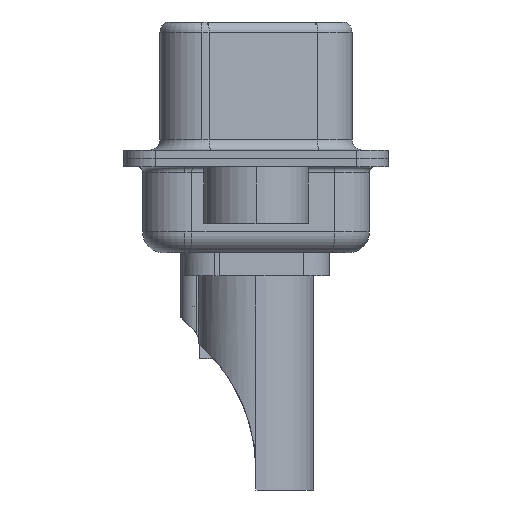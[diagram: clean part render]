
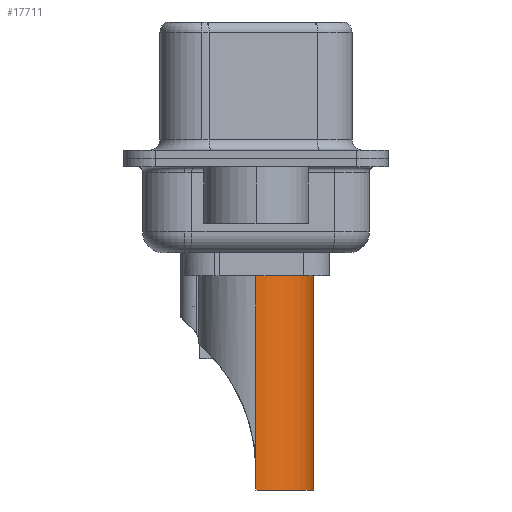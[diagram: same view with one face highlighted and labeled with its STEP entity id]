
A CAD part, left-side view. The second image highlights one B-rep face of the part: STEP entity #17711.
In plain terms, the highlighted cylindrical face has radius 2.75 mm (diameter 5.5 mm), a partial arc.
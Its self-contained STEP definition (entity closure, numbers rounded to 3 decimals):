
#143 = VECTOR ( 'NONE', #11961, 1000. ) ;
#347 = LINE ( 'NONE', #14707, #5019 ) ;
#400 = CARTESIAN_POINT ( 'NONE',  ( 2.75, 0., -8.7 ) ) ;
#703 = VECTOR ( 'NONE', #10427, 1000. ) ;
#766 = CARTESIAN_POINT ( 'NONE',  ( 2.75, 0., 1.5 ) ) ;
#983 = CARTESIAN_POINT ( 'NONE',  ( -2.75, 0., -8.7 ) ) ;
#1158 = CARTESIAN_POINT ( 'NONE',  ( -2.75, 0., 1.5 ) ) ;
#1320 = CARTESIAN_POINT ( 'NONE',  ( 2.75, 0., -7.764 ) ) ;
#1460 = DIRECTION ( 'NONE',  ( 1., 0., 0. ) ) ;
#2112 = VERTEX_POINT ( 'NONE', #766 ) ;
#2835 = VERTEX_POINT ( 'NONE', #983 ) ;
#2941 = LINE ( 'NONE', #4782, #13499 ) ;
#3705 = CYLINDRICAL_SURFACE ( 'NONE', #5382, 2.75 ) ;
#4361 = DIRECTION ( 'NONE',  ( 0., 0., 1. ) ) ;
#4432 = EDGE_CURVE ( 'NONE', #7291, #6750, #2941, .T. ) ;
#4666 = EDGE_LOOP ( 'NONE', ( #12936, #16981, #7817, #22954, #9987, #7148 ) ) ;
#4782 = CARTESIAN_POINT ( 'NONE',  ( -2.75, 0., 4.234 ) ) ;
#5019 = VECTOR ( 'NONE', #15666, 1000. ) ;
#5382 = AXIS2_PLACEMENT_3D ( 'NONE', #5420, #9439, #1460 ) ;
#5420 = CARTESIAN_POINT ( 'NONE',  ( 0., 0., 4.234 ) ) ;
#5637 = EDGE_CURVE ( 'NONE', #13621, #2112, #347, .T. ) ;
#6750 = VERTEX_POINT ( 'NONE', #1158 ) ;
#6873 = VERTEX_POINT ( 'NONE', #10618 ) ;
#6878 = DIRECTION ( 'NONE',  ( 0., 0., 1. ) ) ;
#7148 = ORIENTED_EDGE ( 'NONE', *, *, #16352, .F. ) ;
#7291 = VERTEX_POINT ( 'NONE', #15715 ) ;
#7748 = AXIS2_PLACEMENT_3D ( 'NONE', #9048, #22856, #11063 ) ;
#7817 = ORIENTED_EDGE ( 'NONE', *, *, #8348, .T. ) ;
#8348 = EDGE_CURVE ( 'NONE', #2835, #6873, #8665, .T. ) ;
#8665 = CIRCLE ( 'NONE', #7748, 2.75 ) ;
#9048 = CARTESIAN_POINT ( 'NONE',  ( 0., 0., -8.7 ) ) ;
#9439 = DIRECTION ( 'NONE',  ( 0., 0., 1. ) ) ;
#9971 = CARTESIAN_POINT ( 'NONE',  ( -2.75, 0., -8.7 ) ) ;
#9987 = ORIENTED_EDGE ( 'NONE', *, *, #5637, .T. ) ;
#10162 = EDGE_CURVE ( 'NONE', #7291, #2835, #16049, .T. ) ;
#10427 = DIRECTION ( 'NONE',  ( 0., 0., -1. ) ) ;
#10618 = CARTESIAN_POINT ( 'NONE',  ( 2.75, 0., -8.7 ) ) ;
#11063 = DIRECTION ( 'NONE',  ( 1., 0., 0. ) ) ;
#11961 = DIRECTION ( 'NONE',  ( 0., 0., -1. ) ) ;
#12936 = ORIENTED_EDGE ( 'NONE', *, *, #4432, .F. ) ;
#13499 = VECTOR ( 'NONE', #4361, 1000. ) ;
#13621 = VERTEX_POINT ( 'NONE', #1320 ) ;
#14707 = CARTESIAN_POINT ( 'NONE',  ( 2.75, 0., 4.234 ) ) ;
#15016 = EDGE_CURVE ( 'NONE', #13621, #6873, #16605, .T. ) ;
#15666 = DIRECTION ( 'NONE',  ( 0., 0., 1. ) ) ;
#15715 = CARTESIAN_POINT ( 'NONE',  ( -2.75, 0., -7.764 ) ) ;
#16049 = LINE ( 'NONE', #9971, #143 ) ;
#16352 = EDGE_CURVE ( 'NONE', #6750, #2112, #19904, .T. ) ;
#16605 = LINE ( 'NONE', #400, #703 ) ;
#16981 = ORIENTED_EDGE ( 'NONE', *, *, #10162, .T. ) ;
#17711 = ADVANCED_FACE ( 'NONE', ( #24757 ), #3705, .T. ) ;
#18779 = CARTESIAN_POINT ( 'NONE',  ( 0., 0., 1.5 ) ) ;
#19904 = CIRCLE ( 'NONE', #22581, 2.75 ) ;
#20740 = DIRECTION ( 'NONE',  ( 1., 0., 0. ) ) ;
#22581 = AXIS2_PLACEMENT_3D ( 'NONE', #18779, #6878, #20740 ) ;
#22856 = DIRECTION ( 'NONE',  ( 0., 0., 1. ) ) ;
#22954 = ORIENTED_EDGE ( 'NONE', *, *, #15016, .F. ) ;
#24757 = FACE_OUTER_BOUND ( 'NONE', #4666, .T. ) ;
